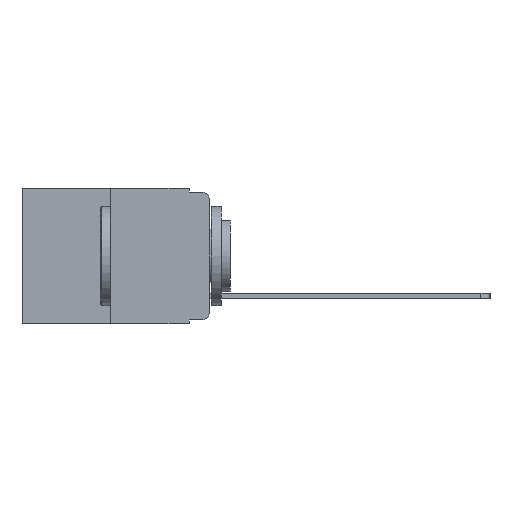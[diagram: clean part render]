
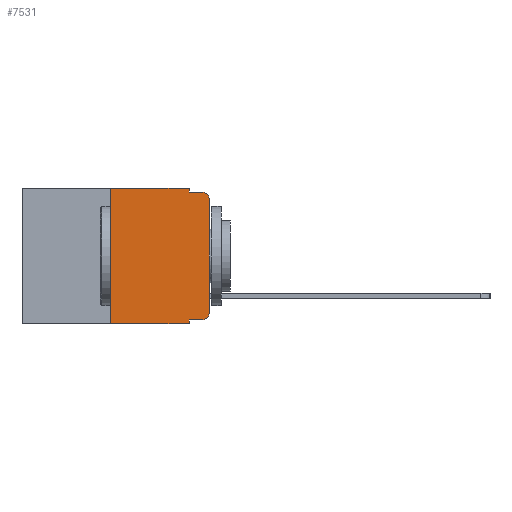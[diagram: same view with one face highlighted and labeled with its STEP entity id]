
A CAD part, left-side view. The second image highlights one B-rep face of the part: STEP entity #7531.
In plain terms, the highlighted planar face has unit normal (-1, 0, 0).
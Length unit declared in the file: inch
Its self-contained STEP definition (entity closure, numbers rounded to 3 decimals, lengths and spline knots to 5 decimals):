
#21 = ORIENTED_EDGE ( 'NONE', *, *, #4647, .F. ) ;
#120 = EDGE_CURVE ( 'NONE', #7548, #1718, #12192, .T. ) ;
#137 = ORIENTED_EDGE ( 'NONE', *, *, #11770, .F. ) ;
#227 = ORIENTED_EDGE ( 'NONE', *, *, #4544, .T. ) ;
#605 = FACE_OUTER_BOUND ( 'NONE', #11834, .T. ) ;
#831 = DIRECTION ( 'NONE',  ( 0., 0., 1. ) ) ;
#913 = ORIENTED_EDGE ( 'NONE', *, *, #11773, .F. ) ;
#1005 = CARTESIAN_POINT ( 'NONE',  ( 0., 0.051, -0.01 ) ) ;
#1222 = VECTOR ( 'NONE', #7459, 39.37008 ) ;
#1366 = ORIENTED_EDGE ( 'NONE', *, *, #11849, .T. ) ;
#1711 = CARTESIAN_POINT ( 'NONE',  ( 0., 0.473, -0.343 ) ) ;
#1718 = VERTEX_POINT ( 'NONE', #11391 ) ;
#1745 = CARTESIAN_POINT ( 'NONE',  ( 0., 0., -0.03 ) ) ;
#2101 = ORIENTED_EDGE ( 'NONE', *, *, #11883, .T. ) ;
#2190 = PLANE ( 'NONE',  #9259 ) ;
#2620 = VERTEX_POINT ( 'NONE', #3485 ) ;
#2627 = VERTEX_POINT ( 'NONE', #8865 ) ;
#2665 = VECTOR ( 'NONE', #12164, 39.37008 ) ;
#3247 = CARTESIAN_POINT ( 'NONE',  ( 0., 0., -0.313 ) ) ;
#3367 = ORIENTED_EDGE ( 'NONE', *, *, #5180, .T. ) ;
#3389 = CARTESIAN_POINT ( 'NONE',  ( 0., 0.051, 0. ) ) ;
#3430 = DIRECTION ( 'NONE',  ( -1., 0., 0. ) ) ;
#3485 = CARTESIAN_POINT ( 'NONE',  ( 0., 0.051, 0. ) ) ;
#3569 = ORIENTED_EDGE ( 'NONE', *, *, #4668, .F. ) ;
#3669 = VERTEX_POINT ( 'NONE', #7207 ) ;
#4042 = CARTESIAN_POINT ( 'NONE',  ( 0., 0.051, -0.333 ) ) ;
#4110 = LINE ( 'NONE', #10728, #11268 ) ;
#4544 = EDGE_CURVE ( 'NONE', #2627, #7060, #7995, .T. ) ;
#4583 = DIRECTION ( 'NONE',  ( 1., 0., 0. ) ) ;
#4647 = EDGE_CURVE ( 'NONE', #3669, #2620, #10651, .T. ) ;
#4668 = EDGE_CURVE ( 'NONE', #2620, #7548, #8128, .T. ) ;
#4872 = AXIS2_PLACEMENT_3D ( 'NONE', #11807, #6648, #5833 ) ;
#5156 = VECTOR ( 'NONE', #8937, 39.37008 ) ;
#5180 = EDGE_CURVE ( 'NONE', #6403, #5491, #8920, .T. ) ;
#5186 = EDGE_CURVE ( 'NONE', #5491, #1718, #8650, .T. ) ;
#5193 = ORIENTED_EDGE ( 'NONE', *, *, #5186, .T. ) ;
#5272 = CARTESIAN_POINT ( 'NONE',  ( 0., 0.051, -0.343 ) ) ;
#5491 = VERTEX_POINT ( 'NONE', #1745 ) ;
#5833 = DIRECTION ( 'NONE',  ( 0., 0., -1. ) ) ;
#5835 = VECTOR ( 'NONE', #7384, 39.37008 ) ;
#6403 = VERTEX_POINT ( 'NONE', #3247 ) ;
#6648 = DIRECTION ( 'NONE',  ( -1., 0., 0. ) ) ;
#7060 = VERTEX_POINT ( 'NONE', #5272 ) ;
#7207 = CARTESIAN_POINT ( 'NONE',  ( 0., 0.25, 0. ) ) ;
#7384 = DIRECTION ( 'NONE',  ( 0., 0., -1. ) ) ;
#7459 = DIRECTION ( 'NONE',  ( 0., 0., 1. ) ) ;
#7531 = ADVANCED_FACE ( 'NONE', ( #605 ), #2190, .F. ) ;
#7548 = VERTEX_POINT ( 'NONE', #1005 ) ;
#7791 = LINE ( 'NONE', #12405, #9792 ) ;
#7995 = LINE ( 'NONE', #1711, #2665 ) ;
#8003 = VERTEX_POINT ( 'NONE', #9479 ) ;
#8065 = DIRECTION ( 'NONE',  ( 0., -1., 0. ) ) ;
#8101 = CARTESIAN_POINT ( 'NONE',  ( 0., 0.051, 0. ) ) ;
#8128 = LINE ( 'NONE', #3389, #5835 ) ;
#8336 = VERTEX_POINT ( 'NONE', #4042 ) ;
#8381 = VECTOR ( 'NONE', #8065, 39.37008 ) ;
#8438 = CIRCLE ( 'NONE', #10769, 0.02 ) ;
#8650 = CIRCLE ( 'NONE', #4872, 0.02 ) ;
#8865 = CARTESIAN_POINT ( 'NONE',  ( 0., 0.25, -0.343 ) ) ;
#8920 = LINE ( 'NONE', #9989, #1222 ) ;
#8937 = DIRECTION ( 'NONE',  ( 0., 0., -1. ) ) ;
#9083 = CARTESIAN_POINT ( 'NONE',  ( 0., 0.02, -0.313 ) ) ;
#9259 = AXIS2_PLACEMENT_3D ( 'NONE', #9921, #4583, #10768 ) ;
#9479 = CARTESIAN_POINT ( 'NONE',  ( 0., 0.02, -0.333 ) ) ;
#9792 = VECTOR ( 'NONE', #831, 39.37008 ) ;
#9813 = ORIENTED_EDGE ( 'NONE', *, *, #120, .F. ) ;
#9921 = CARTESIAN_POINT ( 'NONE',  ( 0., 0.473, 0. ) ) ;
#9955 = DIRECTION ( 'NONE',  ( 0., 0., -1. ) ) ;
#9989 = CARTESIAN_POINT ( 'NONE',  ( 0., 0., 0. ) ) ;
#10109 = VECTOR ( 'NONE', #10120, 39.37008 ) ;
#10120 = DIRECTION ( 'NONE',  ( 0., -1., 0. ) ) ;
#10651 = LINE ( 'NONE', #11487, #8381 ) ;
#10728 = CARTESIAN_POINT ( 'NONE',  ( 0., 0.051, -0.333 ) ) ;
#10768 = DIRECTION ( 'NONE',  ( 0., 0., -1. ) ) ;
#10769 = AXIS2_PLACEMENT_3D ( 'NONE', #9083, #3430, #9955 ) ;
#11268 = VECTOR ( 'NONE', #12481, 39.37008 ) ;
#11391 = CARTESIAN_POINT ( 'NONE',  ( 0., 0.02, -0.01 ) ) ;
#11487 = CARTESIAN_POINT ( 'NONE',  ( 0., 0.473, 0. ) ) ;
#11770 = EDGE_CURVE ( 'NONE', #2627, #3669, #7791, .T. ) ;
#11773 = EDGE_CURVE ( 'NONE', #8336, #7060, #12136, .T. ) ;
#11807 = CARTESIAN_POINT ( 'NONE',  ( 0., 0.02, -0.03 ) ) ;
#11834 = EDGE_LOOP ( 'NONE', ( #3367, #5193, #9813, #3569, #21, #137, #227, #913, #1366, #2101 ) ) ;
#11849 = EDGE_CURVE ( 'NONE', #8336, #8003, #4110, .T. ) ;
#11879 = CARTESIAN_POINT ( 'NONE',  ( 0., 0.051, -0.01 ) ) ;
#11883 = EDGE_CURVE ( 'NONE', #8003, #6403, #8438, .T. ) ;
#12136 = LINE ( 'NONE', #8101, #5156 ) ;
#12164 = DIRECTION ( 'NONE',  ( 0., -1., 0. ) ) ;
#12192 = LINE ( 'NONE', #11879, #10109 ) ;
#12405 = CARTESIAN_POINT ( 'NONE',  ( 0., 0.25, 0. ) ) ;
#12481 = DIRECTION ( 'NONE',  ( 0., -1., 0. ) ) ;
